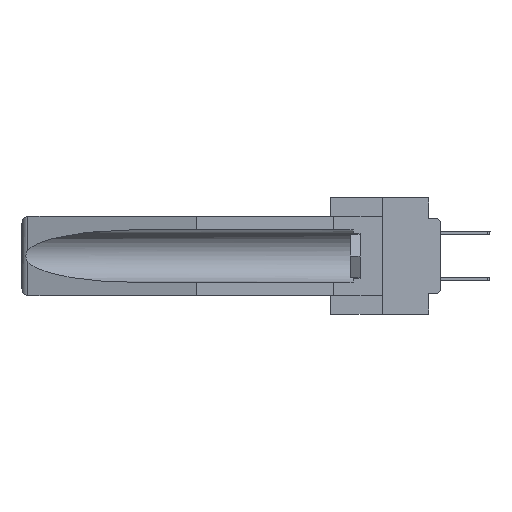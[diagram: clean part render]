
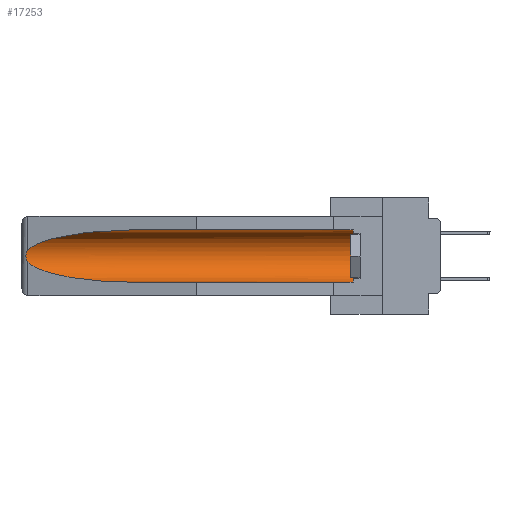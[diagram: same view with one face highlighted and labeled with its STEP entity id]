
A CAD part, left-side view. The second image highlights one B-rep face of the part: STEP entity #17253.
In plain terms, the highlighted cylindrical face has radius 2.857 mm (diameter 5.715 mm), a partial arc.
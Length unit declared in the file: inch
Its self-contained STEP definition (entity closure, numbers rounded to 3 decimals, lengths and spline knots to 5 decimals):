
#418 = LINE ( 'NONE', #12645, #4024 ) ;
#451 = VERTEX_POINT ( 'NONE', #6007 ) ;
#822 = EDGE_CURVE ( 'NONE', #27119, #5169, #10348, .T. ) ;
#828 = ORIENTED_EDGE ( 'NONE', *, *, #16234, .F. ) ;
#1361 = CARTESIAN_POINT ( 'NONE',  ( 0.2675, 1.53308, -0.16763 ) ) ;
#1522 = CARTESIAN_POINT ( 'NONE',  ( 0.26655, 1.53094, -0.18657 ) ) ;
#1684 = CARTESIAN_POINT ( 'NONE',  ( 0.26597, 1.5296, -0.19026 ) ) ;
#2448 =( BOUNDED_CURVE ( )  B_SPLINE_CURVE ( 3, ( #8780, #28887, #28276, #14322 ),
 .UNSPECIFIED., .F., .F. ) 
 B_SPLINE_CURVE_WITH_KNOTS ( ( 4, 4 ),
 ( 0.1948, 1.5708 ),
 .UNSPECIFIED. ) 
 CURVE ( )  GEOMETRIC_REPRESENTATION_ITEM ( )  RATIONAL_B_SPLINE_CURVE ( ( 1., 0.848, 0.848, 1. ) ) 
 REPRESENTATION_ITEM ( '' )  );
#3300 = CARTESIAN_POINT ( 'NONE',  ( 0.155, 0.126, -0.1715 ) ) ;
#4024 = VECTOR ( 'NONE', #22312, 39.37008 ) ;
#4257 = ORIENTED_EDGE ( 'NONE', *, *, #822, .T. ) ;
#5169 = VERTEX_POINT ( 'NONE', #8439 ) ;
#5390 = CARTESIAN_POINT ( 'NONE',  ( 0.26537, 1.52718, -0.14972 ) ) ;
#5588 = DIRECTION ( 'NONE',  ( 0., 0., 1. ) ) ;
#5649 = ORIENTED_EDGE ( 'NONE', *, *, #12507, .T. ) ;
#5947 = CARTESIAN_POINT ( 'NONE',  ( 0.155, 1.07973, -0.059 ) ) ;
#5972 = CARTESIAN_POINT ( 'NONE',  ( 0.26537, 1.52718, -0.19328 ) ) ;
#6007 = CARTESIAN_POINT ( 'NONE',  ( 0.155, 1.07973, -0.284 ) ) ;
#6067 = LINE ( 'NONE', #15746, #24577 ) ;
#7020 = ORIENTED_EDGE ( 'NONE', *, *, #30528, .T. ) ;
#7830 = EDGE_LOOP ( 'NONE', ( #7020, #4257, #18526, #828, #5649, #8990 ) ) ;
#8129 = VERTEX_POINT ( 'NONE', #24894 ) ;
#8439 = CARTESIAN_POINT ( 'NONE',  ( 0.26537, 1.52718, -0.19328 ) ) ;
#8780 = CARTESIAN_POINT ( 'NONE',  ( 0.26537, 1.52718, -0.19328 ) ) ;
#8990 = ORIENTED_EDGE ( 'NONE', *, *, #24957, .T. ) ;
#10348 = B_SPLINE_CURVE_WITH_KNOTS ( 'NONE', 3,
 ( #15651, #13586, #25467, #30244, #1361, #11364, #13428, #1522, #1684, #5972 ),
 .UNSPECIFIED., .F., .F.,
 ( 4, 2, 2, 2, 4 ),
 ( 0., 0.00029, 0.00058, 0.00087, 0.00117 ),
 .UNSPECIFIED. ) ;
#10445 = CIRCLE ( 'NONE', #26121, 0.1125 ) ;
#11364 = CARTESIAN_POINT ( 'NONE',  ( 0.2675, 1.53308, -0.17534 ) ) ;
#12507 = EDGE_CURVE ( 'NONE', #19835, #8129, #10445, .T. ) ;
#12572 = FACE_OUTER_BOUND ( 'NONE', #7830, .T. ) ;
#12645 = CARTESIAN_POINT ( 'NONE',  ( 0.155, -0.30754, -0.284 ) ) ;
#13146 = DIRECTION ( 'NONE',  ( 0., 0., 1. ) ) ;
#13328 = CARTESIAN_POINT ( 'NONE',  ( 0.155, 0.126, -0.284 ) ) ;
#13428 = CARTESIAN_POINT ( 'NONE',  ( 0.2673, 1.53269, -0.17917 ) ) ;
#13586 = CARTESIAN_POINT ( 'NONE',  ( 0.26597, 1.52961, -0.15275 ) ) ;
#14322 = CARTESIAN_POINT ( 'NONE',  ( 0.155, 1.07973, -0.284 ) ) ;
#14959 = CARTESIAN_POINT ( 'NONE',  ( 0.155, -0.30754, -0.1715 ) ) ;
#15651 = CARTESIAN_POINT ( 'NONE',  ( 0.26537, 1.52718, -0.14972 ) ) ;
#15746 = CARTESIAN_POINT ( 'NONE',  ( 0.155, -0.30754, -0.059 ) ) ;
#15836 = DIRECTION ( 'NONE',  ( 0., -1., 0. ) ) ;
#16234 = EDGE_CURVE ( 'NONE', #19835, #451, #418, .T. ) ;
#17253 = ADVANCED_FACE ( 'NONE', ( #12572 ), #27149, .F. ) ;
#17595 = CARTESIAN_POINT ( 'NONE',  ( 0.25451, 1.48313, -0.09465 ) ) ;
#18526 = ORIENTED_EDGE ( 'NONE', *, *, #28418, .T. ) ;
#19835 = VERTEX_POINT ( 'NONE', #13328 ) ;
#20729 = CARTESIAN_POINT ( 'NONE',  ( 0.26537, 1.52718, -0.14972 ) ) ;
#21288 = AXIS2_PLACEMENT_3D ( 'NONE', #14959, #22551, #5588 ) ;
#22312 = DIRECTION ( 'NONE',  ( 0., 1., 0. ) ) ;
#22551 = DIRECTION ( 'NONE',  ( 0., 1., 0. ) ) ;
#24253 = CARTESIAN_POINT ( 'NONE',  ( 0.155, 1.07973, -0.059 ) ) ;
#24378 = VERTEX_POINT ( 'NONE', #5947 ) ;
#24577 = VECTOR ( 'NONE', #30344, 39.37008 ) ;
#24894 = CARTESIAN_POINT ( 'NONE',  ( 0.155, 0.126, -0.059 ) ) ;
#24957 = EDGE_CURVE ( 'NONE', #8129, #24378, #6067, .T. ) ;
#25467 = CARTESIAN_POINT ( 'NONE',  ( 0.26654, 1.53092, -0.15636 ) ) ;
#26121 = AXIS2_PLACEMENT_3D ( 'NONE', #3300, #15836, #13146 ) ;
#26139 =( BOUNDED_CURVE ( )  B_SPLINE_CURVE ( 3, ( #24253, #27111, #17595, #5390 ),
 .UNSPECIFIED., .F., .F. ) 
 B_SPLINE_CURVE_WITH_KNOTS ( ( 4, 4 ),
 ( 4.71239, 6.08839 ),
 .UNSPECIFIED. ) 
 CURVE ( )  GEOMETRIC_REPRESENTATION_ITEM ( )  RATIONAL_B_SPLINE_CURVE ( ( 1., 0.848, 0.848, 1. ) ) 
 REPRESENTATION_ITEM ( '' )  );
#27111 = CARTESIAN_POINT ( 'NONE',  ( 0.21114, 1.30732, -0.059 ) ) ;
#27119 = VERTEX_POINT ( 'NONE', #20729 ) ;
#27149 = CYLINDRICAL_SURFACE ( 'NONE', #21288, 0.1125 ) ;
#28276 = CARTESIAN_POINT ( 'NONE',  ( 0.21114, 1.30732, -0.284 ) ) ;
#28418 = EDGE_CURVE ( 'NONE', #5169, #451, #2448, .T. ) ;
#28887 = CARTESIAN_POINT ( 'NONE',  ( 0.25451, 1.48313, -0.24835 ) ) ;
#30244 = CARTESIAN_POINT ( 'NONE',  ( 0.2673, 1.5327, -0.16383 ) ) ;
#30344 = DIRECTION ( 'NONE',  ( 0., 1., 0. ) ) ;
#30528 = EDGE_CURVE ( 'NONE', #24378, #27119, #26139, .T. ) ;
